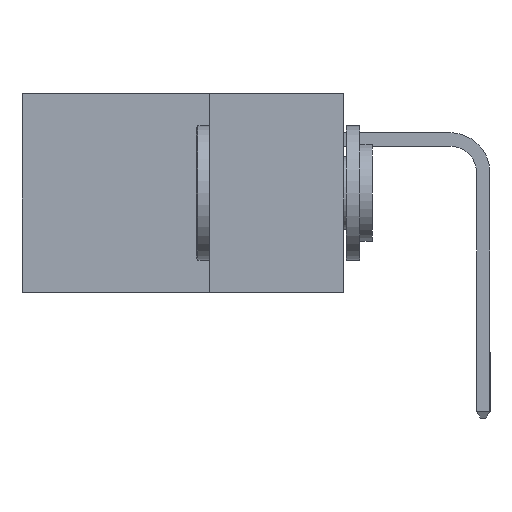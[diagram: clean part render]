
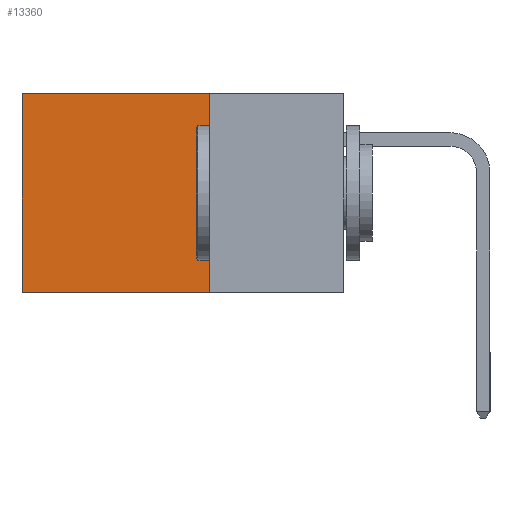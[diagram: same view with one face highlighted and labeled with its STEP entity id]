
A CAD part, left-side view. The second image highlights one B-rep face of the part: STEP entity #13360.
In plain terms, the highlighted planar face has unit normal (-1, 0, 0).
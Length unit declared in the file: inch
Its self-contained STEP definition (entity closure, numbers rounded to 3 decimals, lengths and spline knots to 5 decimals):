
#529 = DIRECTION ( 'NONE',  ( 0., 0., -1. ) ) ;
#734 = LINE ( 'NONE', #8084, #11847 ) ;
#1172 = ORIENTED_EDGE ( 'NONE', *, *, #16458, .T. ) ;
#2321 = DIRECTION ( 'NONE',  ( 0., 0., -1. ) ) ;
#2529 = FACE_OUTER_BOUND ( 'NONE', #17115, .T. ) ;
#2943 = VECTOR ( 'NONE', #2321, 39.37008 ) ;
#4472 = LINE ( 'NONE', #11919, #2943 ) ;
#5110 = DIRECTION ( 'NONE',  ( 0., 0., -1. ) ) ;
#5163 = VECTOR ( 'NONE', #5110, 39.37008 ) ;
#6178 = LINE ( 'NONE', #18117, #5163 ) ;
#6611 = CARTESIAN_POINT ( 'NONE',  ( 0.298, 0.25, -0.37 ) ) ;
#8084 = CARTESIAN_POINT ( 'NONE',  ( 0.298, 0.25, 0. ) ) ;
#8781 = DIRECTION ( 'NONE',  ( 1., 0., 0. ) ) ;
#8989 = VERTEX_POINT ( 'NONE', #11137 ) ;
#9174 = EDGE_CURVE ( 'NONE', #8989, #14610, #10124, .T. ) ;
#10124 = LINE ( 'NONE', #6611, #11144 ) ;
#10682 = CARTESIAN_POINT ( 'NONE',  ( 0.298, 0.6, -0.37 ) ) ;
#10708 = ORIENTED_EDGE ( 'NONE', *, *, #18169, .T. ) ;
#11137 = CARTESIAN_POINT ( 'NONE',  ( 0.298, 0.25, -0.37 ) ) ;
#11139 = CARTESIAN_POINT ( 'NONE',  ( 0.298, 0.6, 0. ) ) ;
#11144 = VECTOR ( 'NONE', #19662, 39.37008 ) ;
#11463 = CARTESIAN_POINT ( 'NONE',  ( 0.298, 0.25, 0. ) ) ;
#11847 = VECTOR ( 'NONE', #17963, 39.37008 ) ;
#11919 = CARTESIAN_POINT ( 'NONE',  ( 0.298, 0.6, 0. ) ) ;
#12326 = CARTESIAN_POINT ( 'NONE',  ( 0.298, 0.25, 0. ) ) ;
#13360 = ADVANCED_FACE ( 'NONE', ( #2529 ), #19540, .F. ) ;
#13525 = VERTEX_POINT ( 'NONE', #12326 ) ;
#14216 = VERTEX_POINT ( 'NONE', #11139 ) ;
#14610 = VERTEX_POINT ( 'NONE', #10682 ) ;
#16458 = EDGE_CURVE ( 'NONE', #14216, #14610, #4472, .T. ) ;
#17115 = EDGE_LOOP ( 'NONE', ( #1172, #20536, #20057, #10708 ) ) ;
#17499 = AXIS2_PLACEMENT_3D ( 'NONE', #11463, #8781, #529 ) ;
#17687 = EDGE_CURVE ( 'NONE', #13525, #8989, #6178, .T. ) ;
#17963 = DIRECTION ( 'NONE',  ( 0., 1., 0. ) ) ;
#18117 = CARTESIAN_POINT ( 'NONE',  ( 0.298, 0.25, 0. ) ) ;
#18169 = EDGE_CURVE ( 'NONE', #13525, #14216, #734, .T. ) ;
#19540 = PLANE ( 'NONE',  #17499 ) ;
#19662 = DIRECTION ( 'NONE',  ( 0., 1., 0. ) ) ;
#20057 = ORIENTED_EDGE ( 'NONE', *, *, #17687, .F. ) ;
#20536 = ORIENTED_EDGE ( 'NONE', *, *, #9174, .F. ) ;
